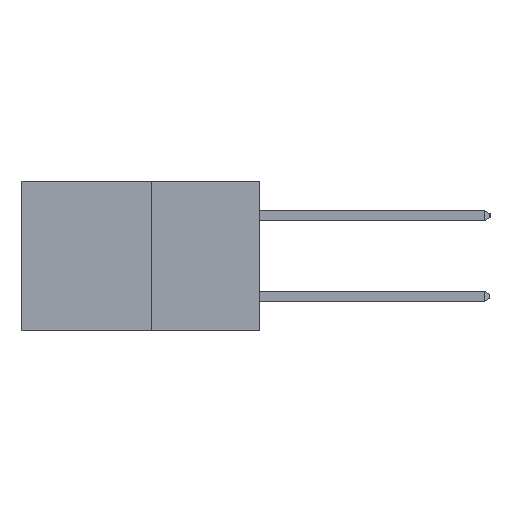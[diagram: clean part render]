
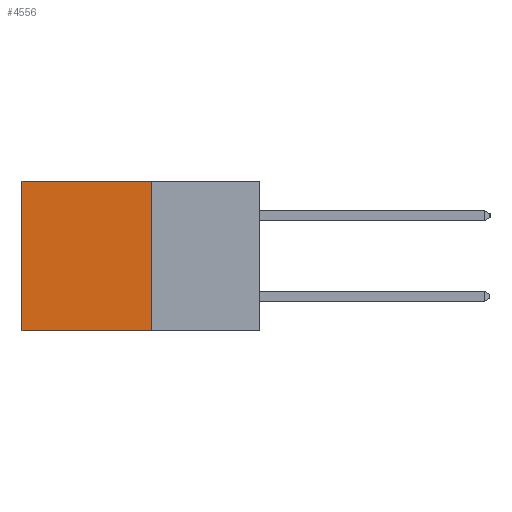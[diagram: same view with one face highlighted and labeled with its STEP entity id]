
A CAD part, left-side view. The second image highlights one B-rep face of the part: STEP entity #4556.
In plain terms, the highlighted planar face has unit normal (-1, 0, 0).
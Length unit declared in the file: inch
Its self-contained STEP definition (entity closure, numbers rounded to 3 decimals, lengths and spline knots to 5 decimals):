
#113 = DIRECTION ( 'NONE',  ( 0., 0., -1. ) ) ;
#127 = CARTESIAN_POINT ( 'NONE',  ( 0.277, 0.59, -0.37 ) ) ;
#174 = AXIS2_PLACEMENT_3D ( 'NONE', #4510, #9063, #9173 ) ;
#851 = CARTESIAN_POINT ( 'NONE',  ( 0.277, 0.27, -0.37 ) ) ;
#1110 = LINE ( 'NONE', #127, #5326 ) ;
#1120 = LINE ( 'NONE', #8483, #9621 ) ;
#1313 = VERTEX_POINT ( 'NONE', #5935 ) ;
#1380 = FACE_OUTER_BOUND ( 'NONE', #10107, .T. ) ;
#1381 = CARTESIAN_POINT ( 'NONE',  ( 0.277, 0.27, 0. ) ) ;
#2134 = CARTESIAN_POINT ( 'NONE',  ( 0.277, 0.27, 0. ) ) ;
#3108 = ORIENTED_EDGE ( 'NONE', *, *, #8700, .F. ) ;
#4014 = EDGE_CURVE ( 'NONE', #7485, #1313, #1120, .T. ) ;
#4114 = LINE ( 'NONE', #2134, #4398 ) ;
#4279 = VERTEX_POINT ( 'NONE', #6823 ) ;
#4398 = VECTOR ( 'NONE', #7159, 39.37008 ) ;
#4510 = CARTESIAN_POINT ( 'NONE',  ( 0.277, 0.27, -0.37 ) ) ;
#4522 = EDGE_CURVE ( 'NONE', #4279, #1313, #1110, .T. ) ;
#4556 = ADVANCED_FACE ( 'NONE', ( #1380 ), #9064, .F. ) ;
#5326 = VECTOR ( 'NONE', #113, 39.37008 ) ;
#5376 = DIRECTION ( 'NONE',  ( 0., 1., 0. ) ) ;
#5935 = CARTESIAN_POINT ( 'NONE',  ( 0.277, 0.59, -0.37 ) ) ;
#6139 = ORIENTED_EDGE ( 'NONE', *, *, #7814, .T. ) ;
#6786 = ORIENTED_EDGE ( 'NONE', *, *, #4014, .F. ) ;
#6823 = CARTESIAN_POINT ( 'NONE',  ( 0.277, 0.59, 0. ) ) ;
#6916 = ORIENTED_EDGE ( 'NONE', *, *, #4522, .T. ) ;
#7159 = DIRECTION ( 'NONE',  ( 0., 1., 0. ) ) ;
#7485 = VERTEX_POINT ( 'NONE', #851 ) ;
#7493 = LINE ( 'NONE', #9737, #9334 ) ;
#7814 = EDGE_CURVE ( 'NONE', #9992, #4279, #4114, .T. ) ;
#8194 = DIRECTION ( 'NONE',  ( 0., 0., -1. ) ) ;
#8483 = CARTESIAN_POINT ( 'NONE',  ( 0.277, 0.27, -0.37 ) ) ;
#8700 = EDGE_CURVE ( 'NONE', #9992, #7485, #7493, .T. ) ;
#9063 = DIRECTION ( 'NONE',  ( 1., 0., 0. ) ) ;
#9064 = PLANE ( 'NONE',  #174 ) ;
#9173 = DIRECTION ( 'NONE',  ( 0., 0., -1. ) ) ;
#9334 = VECTOR ( 'NONE', #8194, 39.37008 ) ;
#9621 = VECTOR ( 'NONE', #5376, 39.37008 ) ;
#9737 = CARTESIAN_POINT ( 'NONE',  ( 0.277, 0.27, -0.37 ) ) ;
#9992 = VERTEX_POINT ( 'NONE', #1381 ) ;
#10107 = EDGE_LOOP ( 'NONE', ( #6916, #6786, #3108, #6139 ) ) ;
